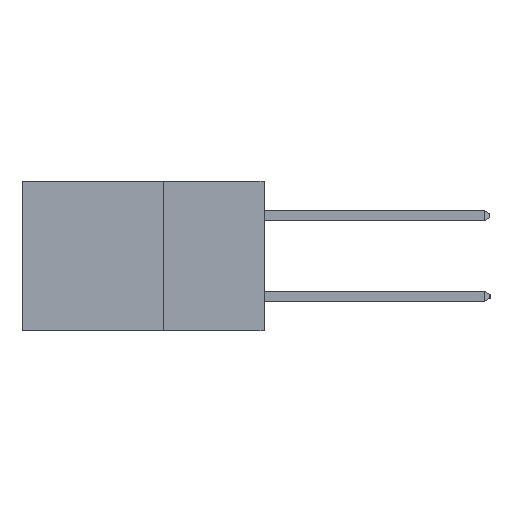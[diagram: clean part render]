
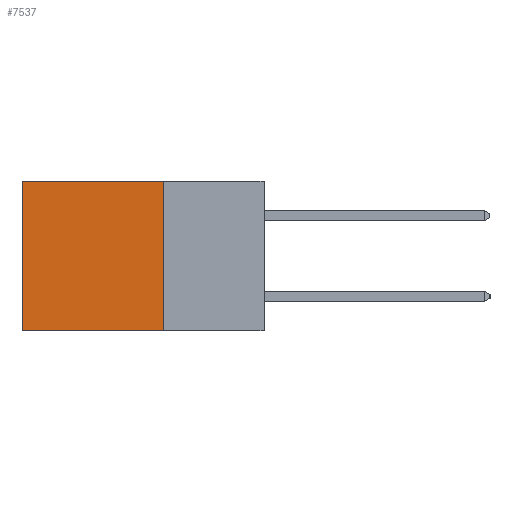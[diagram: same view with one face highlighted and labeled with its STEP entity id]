
A CAD part, left-side view. The second image highlights one B-rep face of the part: STEP entity #7537.
In plain terms, the highlighted planar face has unit normal (-1, 0, 0).
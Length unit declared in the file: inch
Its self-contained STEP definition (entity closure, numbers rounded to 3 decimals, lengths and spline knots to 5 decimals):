
#68 = VERTEX_POINT ( 'NONE', #15400 ) ;
#73 = CARTESIAN_POINT ( 'NONE',  ( 0.2615, 0.6, 0. ) ) ;
#1029 = CARTESIAN_POINT ( 'NONE',  ( 0.2615, 0.6, -0.37 ) ) ;
#1060 = EDGE_CURVE ( 'NONE', #2692, #5517, #6460, .T. ) ;
#1095 = CARTESIAN_POINT ( 'NONE',  ( 0.2615, 0.25, -0.37 ) ) ;
#1104 = VERTEX_POINT ( 'NONE', #9033 ) ;
#1469 = EDGE_CURVE ( 'NONE', #68, #1104, #6436, .T. ) ;
#1531 = VECTOR ( 'NONE', #11886, 39.37008 ) ;
#1954 = LINE ( 'NONE', #1029, #1531 ) ;
#2692 = VERTEX_POINT ( 'NONE', #14458 ) ;
#2877 = DIRECTION ( 'NONE',  ( 0., 0., -1. ) ) ;
#3303 = CARTESIAN_POINT ( 'NONE',  ( 0.2615, 0.25, -0.37 ) ) ;
#4615 = FACE_OUTER_BOUND ( 'NONE', #15790, .T. ) ;
#5517 = VERTEX_POINT ( 'NONE', #73 ) ;
#5528 = ORIENTED_EDGE ( 'NONE', *, *, #1060, .T. ) ;
#5798 = ORIENTED_EDGE ( 'NONE', *, *, #1469, .F. ) ;
#6436 = LINE ( 'NONE', #1095, #16717 ) ;
#6460 = LINE ( 'NONE', #9789, #9610 ) ;
#7537 = ADVANCED_FACE ( 'NONE', ( #4615 ), #8268, .F. ) ;
#7564 = ORIENTED_EDGE ( 'NONE', *, *, #15121, .F. ) ;
#7707 = AXIS2_PLACEMENT_3D ( 'NONE', #9629, #10991, #2877 ) ;
#8268 = PLANE ( 'NONE',  #7707 ) ;
#8692 = DIRECTION ( 'NONE',  ( 0., 0., -1. ) ) ;
#9033 = CARTESIAN_POINT ( 'NONE',  ( 0.2615, 0.6, -0.37 ) ) ;
#9610 = VECTOR ( 'NONE', #10051, 39.37008 ) ;
#9629 = CARTESIAN_POINT ( 'NONE',  ( 0.2615, 0.25, -0.37 ) ) ;
#9789 = CARTESIAN_POINT ( 'NONE',  ( 0.2615, 0.25, 0. ) ) ;
#10051 = DIRECTION ( 'NONE',  ( 0., 1., 0. ) ) ;
#10991 = DIRECTION ( 'NONE',  ( 1., 0., 0. ) ) ;
#11886 = DIRECTION ( 'NONE',  ( 0., 0., -1. ) ) ;
#12531 = VECTOR ( 'NONE', #8692, 39.37008 ) ;
#13219 = DIRECTION ( 'NONE',  ( 0., 1., 0. ) ) ;
#14458 = CARTESIAN_POINT ( 'NONE',  ( 0.2615, 0.25, 0. ) ) ;
#14496 = EDGE_CURVE ( 'NONE', #5517, #1104, #1954, .T. ) ;
#15121 = EDGE_CURVE ( 'NONE', #2692, #68, #15634, .T. ) ;
#15400 = CARTESIAN_POINT ( 'NONE',  ( 0.2615, 0.25, -0.37 ) ) ;
#15634 = LINE ( 'NONE', #3303, #12531 ) ;
#15790 = EDGE_LOOP ( 'NONE', ( #16228, #5798, #7564, #5528 ) ) ;
#16228 = ORIENTED_EDGE ( 'NONE', *, *, #14496, .T. ) ;
#16717 = VECTOR ( 'NONE', #13219, 39.37008 ) ;
